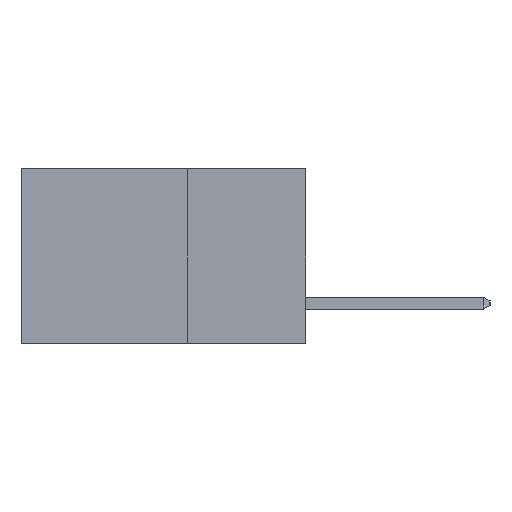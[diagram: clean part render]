
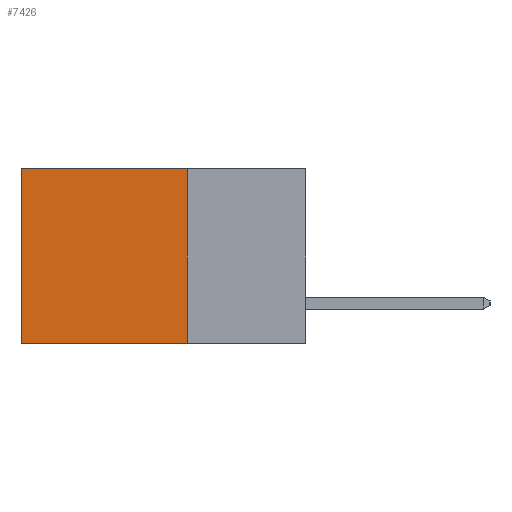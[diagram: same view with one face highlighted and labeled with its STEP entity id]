
A CAD part, left-side view. The second image highlights one B-rep face of the part: STEP entity #7426.
In plain terms, the highlighted planar face has unit normal (-1, 0, 0).
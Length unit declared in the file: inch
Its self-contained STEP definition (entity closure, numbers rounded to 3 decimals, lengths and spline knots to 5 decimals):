
#1018 = VERTEX_POINT ( 'NONE', #16640 ) ;
#1079 = PLANE ( 'NONE',  #5321 ) ;
#1950 = EDGE_CURVE ( 'NONE', #1018, #6550, #13001, .T. ) ;
#2489 = CARTESIAN_POINT ( 'NONE',  ( 0.2615, 0.25, -0.37 ) ) ;
#2993 = ORIENTED_EDGE ( 'NONE', *, *, #11859, .F. ) ;
#3605 = ORIENTED_EDGE ( 'NONE', *, *, #11742, .T. ) ;
#3660 = VERTEX_POINT ( 'NONE', #9974 ) ;
#3731 = VECTOR ( 'NONE', #7565, 39.37008 ) ;
#4878 = ORIENTED_EDGE ( 'NONE', *, *, #14900, .F. ) ;
#5124 = VERTEX_POINT ( 'NONE', #10052 ) ;
#5321 = AXIS2_PLACEMENT_3D ( 'NONE', #2489, #14853, #6765 ) ;
#5384 = DIRECTION ( 'NONE',  ( 0., 0., -1. ) ) ;
#5625 = CARTESIAN_POINT ( 'NONE',  ( 0.2615, 0.25, -0.37 ) ) ;
#6550 = VERTEX_POINT ( 'NONE', #16961 ) ;
#6765 = DIRECTION ( 'NONE',  ( 0., 0., -1. ) ) ;
#7426 = ADVANCED_FACE ( 'NONE', ( #10928 ), #1079, .F. ) ;
#7565 = DIRECTION ( 'NONE',  ( 0., 0., -1. ) ) ;
#7900 = VECTOR ( 'NONE', #15090, 39.37008 ) ;
#8142 = CARTESIAN_POINT ( 'NONE',  ( 0.2615, 0.6, -0.37 ) ) ;
#9185 = LINE ( 'NONE', #5625, #7900 ) ;
#9974 = CARTESIAN_POINT ( 'NONE',  ( 0.2615, 0.25, -0.37 ) ) ;
#10052 = CARTESIAN_POINT ( 'NONE',  ( 0.2615, 0.6, -0.37 ) ) ;
#10204 = ORIENTED_EDGE ( 'NONE', *, *, #1950, .T. ) ;
#10241 = LINE ( 'NONE', #15661, #3731 ) ;
#10928 = FACE_OUTER_BOUND ( 'NONE', #12421, .T. ) ;
#11742 = EDGE_CURVE ( 'NONE', #6550, #5124, #17124, .T. ) ;
#11859 = EDGE_CURVE ( 'NONE', #3660, #5124, #9185, .T. ) ;
#12421 = EDGE_LOOP ( 'NONE', ( #3605, #2993, #4878, #10204 ) ) ;
#13001 = LINE ( 'NONE', #14122, #16963 ) ;
#13192 = DIRECTION ( 'NONE',  ( 0., 1., 0. ) ) ;
#13588 = VECTOR ( 'NONE', #5384, 39.37008 ) ;
#14122 = CARTESIAN_POINT ( 'NONE',  ( 0.2615, 0.25, 0. ) ) ;
#14853 = DIRECTION ( 'NONE',  ( 1., 0., 0. ) ) ;
#14900 = EDGE_CURVE ( 'NONE', #1018, #3660, #10241, .T. ) ;
#15090 = DIRECTION ( 'NONE',  ( 0., 1., 0. ) ) ;
#15661 = CARTESIAN_POINT ( 'NONE',  ( 0.2615, 0.25, -0.37 ) ) ;
#16640 = CARTESIAN_POINT ( 'NONE',  ( 0.2615, 0.25, 0. ) ) ;
#16961 = CARTESIAN_POINT ( 'NONE',  ( 0.2615, 0.6, 0. ) ) ;
#16963 = VECTOR ( 'NONE', #13192, 39.37008 ) ;
#17124 = LINE ( 'NONE', #8142, #13588 ) ;
